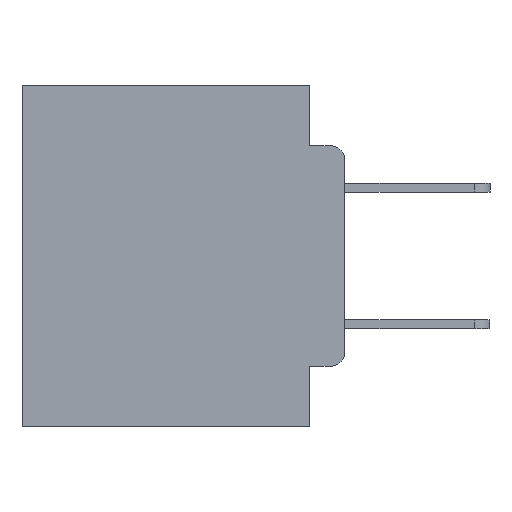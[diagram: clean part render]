
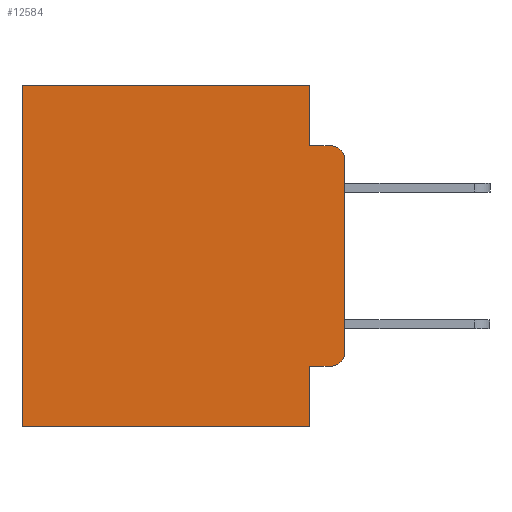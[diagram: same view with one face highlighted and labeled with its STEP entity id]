
A CAD part, left-side view. The second image highlights one B-rep face of the part: STEP entity #12584.
In plain terms, the highlighted planar face has unit normal (-1, 0, 0).
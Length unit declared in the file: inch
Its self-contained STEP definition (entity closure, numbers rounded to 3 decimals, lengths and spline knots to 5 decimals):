
#334 = LINE ( 'NONE', #15743, #27919 ) ;
#737 = EDGE_CURVE ( 'NONE', #6662, #26748, #16056, .T. ) ;
#1090 = CARTESIAN_POINT ( 'NONE',  ( 0.298, 0.051, 0. ) ) ;
#1211 = CARTESIAN_POINT ( 'NONE',  ( 0.298, 0.051, -0.4115 ) ) ;
#1444 = DIRECTION ( 'NONE',  ( 0., 0., -1. ) ) ;
#1494 = DIRECTION ( 'NONE',  ( 0., 0., -1. ) ) ;
#2396 = CARTESIAN_POINT ( 'NONE',  ( 0.298, 0.051, 0. ) ) ;
#2688 = CARTESIAN_POINT ( 'NONE',  ( 0.298, 0.051, -0.5 ) ) ;
#2990 = LINE ( 'NONE', #3947, #19807 ) ;
#3287 = CARTESIAN_POINT ( 'NONE',  ( 0.298, 0.02, -0.4115 ) ) ;
#3379 = VECTOR ( 'NONE', #7772, 39.37008 ) ;
#3387 = EDGE_LOOP ( 'NONE', ( #12811, #12873, #13233, #24694, #13655, #18986, #27216, #21154, #11673, #24519 ) ) ;
#3712 = CARTESIAN_POINT ( 'NONE',  ( 0.298, 0., 0. ) ) ;
#3756 = CARTESIAN_POINT ( 'NONE',  ( 0.298, 0.02, -0.1085 ) ) ;
#3947 = CARTESIAN_POINT ( 'NONE',  ( 0.298, 0.051, -0.4115 ) ) ;
#4601 = CIRCLE ( 'NONE', #5662, 0.02 ) ;
#4660 = CARTESIAN_POINT ( 'NONE',  ( 0.298, 0., 0. ) ) ;
#4960 = DIRECTION ( 'NONE',  ( 0., 0., -1. ) ) ;
#5134 = CARTESIAN_POINT ( 'NONE',  ( 0.298, 0.051, -0.0885 ) ) ;
#5162 = LINE ( 'NONE', #22331, #27498 ) ;
#5420 = LINE ( 'NONE', #1090, #27742 ) ;
#5662 = AXIS2_PLACEMENT_3D ( 'NONE', #27502, #14762, #1444 ) ;
#5936 = DIRECTION ( 'NONE',  ( 0., 0., -1. ) ) ;
#6028 = DIRECTION ( 'NONE',  ( 0., 1., 0. ) ) ;
#6142 = FACE_OUTER_BOUND ( 'NONE', #3387, .T. ) ;
#6662 = VERTEX_POINT ( 'NONE', #2396 ) ;
#6820 = CARTESIAN_POINT ( 'NONE',  ( 0.298, 0.473, -0.5 ) ) ;
#7300 = AXIS2_PLACEMENT_3D ( 'NONE', #3756, #19082, #5936 ) ;
#7627 = AXIS2_PLACEMENT_3D ( 'NONE', #3712, #14817, #1494 ) ;
#7772 = DIRECTION ( 'NONE',  ( 0., 0., -1. ) ) ;
#8337 = VERTEX_POINT ( 'NONE', #10585 ) ;
#8429 = CARTESIAN_POINT ( 'NONE',  ( 0.298, 0., -0.1085 ) ) ;
#8583 = EDGE_CURVE ( 'NONE', #19396, #20300, #5162, .T. ) ;
#9095 = CARTESIAN_POINT ( 'NONE',  ( 0.298, 0.02, -0.0885 ) ) ;
#9183 = DIRECTION ( 'NONE',  ( 0., 0., -1. ) ) ;
#9492 = VECTOR ( 'NONE', #11509, 39.37008 ) ;
#9875 = EDGE_CURVE ( 'NONE', #20300, #24308, #24498, .T. ) ;
#10029 = CARTESIAN_POINT ( 'NONE',  ( 0.298, 0., -0.3915 ) ) ;
#10046 = EDGE_CURVE ( 'NONE', #19396, #10187, #2990, .T. ) ;
#10187 = VERTEX_POINT ( 'NONE', #3287 ) ;
#10585 = CARTESIAN_POINT ( 'NONE',  ( 0.298, 0.051, -0.0885 ) ) ;
#11509 = DIRECTION ( 'NONE',  ( 0., 1., 0. ) ) ;
#11673 = ORIENTED_EDGE ( 'NONE', *, *, #10046, .T. ) ;
#12584 = ADVANCED_FACE ( 'NONE', ( #6142 ), #12594, .F. ) ;
#12594 = PLANE ( 'NONE',  #7627 ) ;
#12811 = ORIENTED_EDGE ( 'NONE', *, *, #24565, .F. ) ;
#12873 = ORIENTED_EDGE ( 'NONE', *, *, #14502, .T. ) ;
#13038 = EDGE_CURVE ( 'NONE', #6662, #8337, #5420, .T. ) ;
#13233 = ORIENTED_EDGE ( 'NONE', *, *, #18828, .F. ) ;
#13655 = ORIENTED_EDGE ( 'NONE', *, *, #737, .T. ) ;
#14353 = CIRCLE ( 'NONE', #7300, 0.02 ) ;
#14502 = EDGE_CURVE ( 'NONE', #22027, #23759, #14353, .T. ) ;
#14762 = DIRECTION ( 'NONE',  ( -1., 0., 0. ) ) ;
#14817 = DIRECTION ( 'NONE',  ( 1., 0., 0. ) ) ;
#14849 = DIRECTION ( 'NONE',  ( 0., -1., 0. ) ) ;
#15154 = LINE ( 'NONE', #22978, #3379 ) ;
#15743 = CARTESIAN_POINT ( 'NONE',  ( 0.298, 0.473, 0. ) ) ;
#15985 = EDGE_CURVE ( 'NONE', #26748, #24308, #334, .T. ) ;
#16056 = LINE ( 'NONE', #4660, #9492 ) ;
#17686 = VERTEX_POINT ( 'NONE', #10029 ) ;
#18300 = DIRECTION ( 'NONE',  ( 0., -1., 0. ) ) ;
#18816 = VECTOR ( 'NONE', #6028, 39.37008 ) ;
#18828 = EDGE_CURVE ( 'NONE', #8337, #23759, #23701, .T. ) ;
#18986 = ORIENTED_EDGE ( 'NONE', *, *, #15985, .T. ) ;
#19082 = DIRECTION ( 'NONE',  ( -1., 0., 0. ) ) ;
#19396 = VERTEX_POINT ( 'NONE', #1211 ) ;
#19807 = VECTOR ( 'NONE', #14849, 39.37008 ) ;
#19947 = CARTESIAN_POINT ( 'NONE',  ( 0.298, 0., -0.5 ) ) ;
#20300 = VERTEX_POINT ( 'NONE', #2688 ) ;
#20335 = CARTESIAN_POINT ( 'NONE',  ( 0.298, 0.473, 0. ) ) ;
#21154 = ORIENTED_EDGE ( 'NONE', *, *, #8583, .F. ) ;
#22027 = VERTEX_POINT ( 'NONE', #8429 ) ;
#22331 = CARTESIAN_POINT ( 'NONE',  ( 0.298, 0.051, 0. ) ) ;
#22363 = VECTOR ( 'NONE', #18300, 39.37008 ) ;
#22978 = CARTESIAN_POINT ( 'NONE',  ( 0.298, 0., 0. ) ) ;
#23033 = DIRECTION ( 'NONE',  ( 0., 0., -1. ) ) ;
#23701 = LINE ( 'NONE', #5134, #22363 ) ;
#23759 = VERTEX_POINT ( 'NONE', #9095 ) ;
#24308 = VERTEX_POINT ( 'NONE', #6820 ) ;
#24498 = LINE ( 'NONE', #19947, #18816 ) ;
#24519 = ORIENTED_EDGE ( 'NONE', *, *, #27492, .T. ) ;
#24565 = EDGE_CURVE ( 'NONE', #22027, #17686, #15154, .T. ) ;
#24694 = ORIENTED_EDGE ( 'NONE', *, *, #13038, .F. ) ;
#26748 = VERTEX_POINT ( 'NONE', #20335 ) ;
#27216 = ORIENTED_EDGE ( 'NONE', *, *, #9875, .F. ) ;
#27492 = EDGE_CURVE ( 'NONE', #10187, #17686, #4601, .T. ) ;
#27498 = VECTOR ( 'NONE', #4960, 39.37008 ) ;
#27502 = CARTESIAN_POINT ( 'NONE',  ( 0.298, 0.02, -0.3915 ) ) ;
#27742 = VECTOR ( 'NONE', #23033, 39.37008 ) ;
#27919 = VECTOR ( 'NONE', #9183, 39.37008 ) ;
